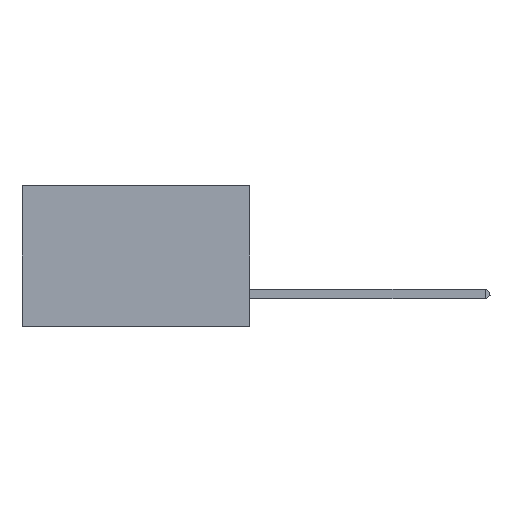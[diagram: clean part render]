
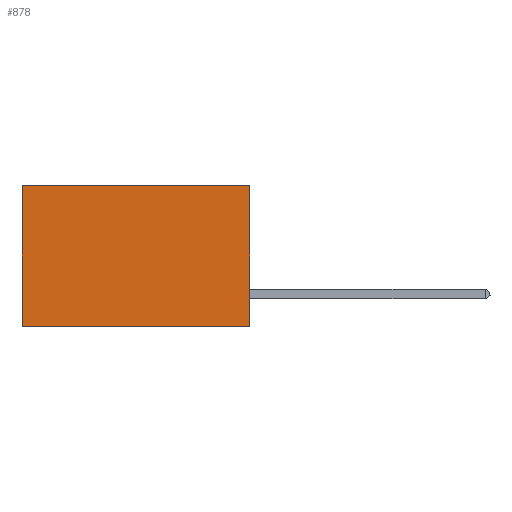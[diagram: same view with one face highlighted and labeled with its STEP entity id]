
A CAD part, left-side view. The second image highlights one B-rep face of the part: STEP entity #878.
In plain terms, the highlighted planar face has unit normal (-1, 0, 0).
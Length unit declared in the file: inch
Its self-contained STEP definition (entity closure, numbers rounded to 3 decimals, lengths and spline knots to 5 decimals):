
#225 = CARTESIAN_POINT ( 'NONE',  ( 0.2875, 0., 0. ) ) ;
#878 = ADVANCED_FACE ( 'NONE', ( #10499 ), #16511, .F. ) ;
#2030 = VECTOR ( 'NONE', #7650, 39.37008 ) ;
#3023 = CARTESIAN_POINT ( 'NONE',  ( 0.2875, 0., -0.37 ) ) ;
#3027 = ORIENTED_EDGE ( 'NONE', *, *, #4902, .T. ) ;
#3036 = VERTEX_POINT ( 'NONE', #3023 ) ;
#3409 = ORIENTED_EDGE ( 'NONE', *, *, #19497, .T. ) ;
#3967 = LINE ( 'NONE', #23313, #22528 ) ;
#4902 = EDGE_CURVE ( 'NONE', #24640, #17114, #26310, .T. ) ;
#5732 = DIRECTION ( 'NONE',  ( 0., 0., -1. ) ) ;
#7413 = CARTESIAN_POINT ( 'NONE',  ( 0.2875, 0.6, 0. ) ) ;
#7650 = DIRECTION ( 'NONE',  ( 0., 0., -1. ) ) ;
#8255 = CARTESIAN_POINT ( 'NONE',  ( 0.2875, 0., 0. ) ) ;
#9170 = EDGE_CURVE ( 'NONE', #14880, #3036, #28575, .T. ) ;
#10499 = FACE_OUTER_BOUND ( 'NONE', #19206, .T. ) ;
#12193 = VECTOR ( 'NONE', #5732, 39.37008 ) ;
#12818 = DIRECTION ( 'NONE',  ( 0., 1., 0. ) ) ;
#13245 = CARTESIAN_POINT ( 'NONE',  ( 0.2875, 0., 0. ) ) ;
#13780 = DIRECTION ( 'NONE',  ( 1., 0., 0. ) ) ;
#14880 = VERTEX_POINT ( 'NONE', #13245 ) ;
#16511 = PLANE ( 'NONE',  #27790 ) ;
#16673 = DIRECTION ( 'NONE',  ( 0., 0., -1. ) ) ;
#16715 = CARTESIAN_POINT ( 'NONE',  ( 0.2875, 0.6, 0. ) ) ;
#17035 = EDGE_CURVE ( 'NONE', #3036, #17114, #3967, .T. ) ;
#17047 = VECTOR ( 'NONE', #21476, 39.37008 ) ;
#17114 = VERTEX_POINT ( 'NONE', #29399 ) ;
#17771 = LINE ( 'NONE', #225, #17047 ) ;
#19077 = ORIENTED_EDGE ( 'NONE', *, *, #17035, .F. ) ;
#19206 = EDGE_LOOP ( 'NONE', ( #3027, #19077, #23159, #3409 ) ) ;
#19497 = EDGE_CURVE ( 'NONE', #14880, #24640, #17771, .T. ) ;
#21476 = DIRECTION ( 'NONE',  ( 0., 1., 0. ) ) ;
#22528 = VECTOR ( 'NONE', #12818, 39.37008 ) ;
#23159 = ORIENTED_EDGE ( 'NONE', *, *, #9170, .F. ) ;
#23313 = CARTESIAN_POINT ( 'NONE',  ( 0.2875, 0., -0.37 ) ) ;
#24640 = VERTEX_POINT ( 'NONE', #7413 ) ;
#25166 = CARTESIAN_POINT ( 'NONE',  ( 0.2875, 0., 0. ) ) ;
#26310 = LINE ( 'NONE', #16715, #2030 ) ;
#27790 = AXIS2_PLACEMENT_3D ( 'NONE', #25166, #13780, #16673 ) ;
#28575 = LINE ( 'NONE', #8255, #12193 ) ;
#29399 = CARTESIAN_POINT ( 'NONE',  ( 0.2875, 0.6, -0.37 ) ) ;
